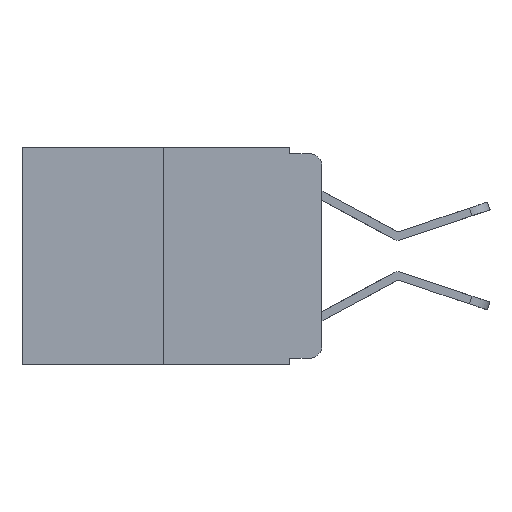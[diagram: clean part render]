
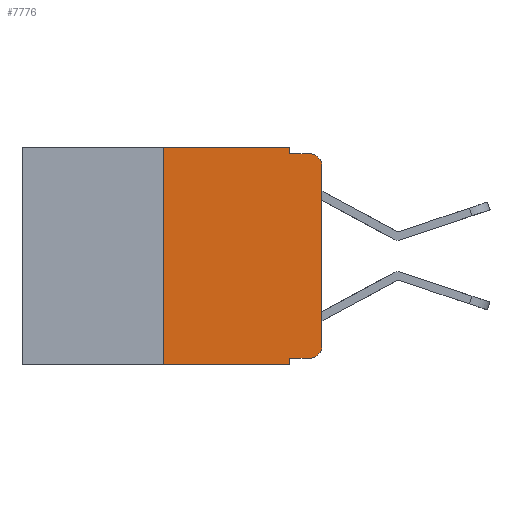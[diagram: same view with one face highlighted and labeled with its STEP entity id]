
A CAD part, left-side view. The second image highlights one B-rep face of the part: STEP entity #7776.
In plain terms, the highlighted planar face has unit normal (-1, 0, 0).
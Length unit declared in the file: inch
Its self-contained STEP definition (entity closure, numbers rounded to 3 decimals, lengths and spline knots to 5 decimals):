
#4 = DIRECTION ( 'NONE',  ( 0., 0., -1. ) ) ;
#167 = ORIENTED_EDGE ( 'NONE', *, *, #11082, .F. ) ;
#398 = CARTESIAN_POINT ( 'NONE',  ( 0., 0.051, 0. ) ) ;
#600 = VERTEX_POINT ( 'NONE', #7231 ) ;
#603 = CARTESIAN_POINT ( 'NONE',  ( 0., 0.473, 0. ) ) ;
#617 = CARTESIAN_POINT ( 'NONE',  ( 0., 0.25, -0.343 ) ) ;
#632 = VECTOR ( 'NONE', #6622, 39.37008 ) ;
#697 = ORIENTED_EDGE ( 'NONE', *, *, #9980, .F. ) ;
#709 = EDGE_CURVE ( 'NONE', #600, #5956, #1566, .T. ) ;
#1296 = CARTESIAN_POINT ( 'NONE',  ( 0., 0.051, -0.333 ) ) ;
#1396 = LINE ( 'NONE', #5989, #6309 ) ;
#1516 = VECTOR ( 'NONE', #7688, 39.37008 ) ;
#1566 = CIRCLE ( 'NONE', #11200, 0.02 ) ;
#1729 = LINE ( 'NONE', #7866, #11044 ) ;
#1887 = AXIS2_PLACEMENT_3D ( 'NONE', #603, #4783, #11041 ) ;
#2132 = AXIS2_PLACEMENT_3D ( 'NONE', #11404, #6099, #4 ) ;
#2157 = DIRECTION ( 'NONE',  ( 0., 0., -1. ) ) ;
#2173 = EDGE_CURVE ( 'NONE', #11813, #600, #6433, .T. ) ;
#2207 = LINE ( 'NONE', #9805, #11421 ) ;
#2435 = CARTESIAN_POINT ( 'NONE',  ( 0., 0.25, 0. ) ) ;
#2783 = CARTESIAN_POINT ( 'NONE',  ( 0., 0.473, 0. ) ) ;
#2790 = PLANE ( 'NONE',  #1887 ) ;
#2823 = EDGE_LOOP ( 'NONE', ( #3531, #11302, #6900, #167, #8032, #11444, #7324, #697, #4766, #12078 ) ) ;
#3334 = DIRECTION ( 'NONE',  ( 0., 0., -1. ) ) ;
#3367 = VERTEX_POINT ( 'NONE', #617 ) ;
#3529 = DIRECTION ( 'NONE',  ( 0., 0., -1. ) ) ;
#3531 = ORIENTED_EDGE ( 'NONE', *, *, #2173, .T. ) ;
#3745 = VERTEX_POINT ( 'NONE', #5617 ) ;
#3793 = LINE ( 'NONE', #2783, #632 ) ;
#4589 = VERTEX_POINT ( 'NONE', #6324 ) ;
#4712 = VERTEX_POINT ( 'NONE', #2435 ) ;
#4766 = ORIENTED_EDGE ( 'NONE', *, *, #8767, .T. ) ;
#4783 = DIRECTION ( 'NONE',  ( 1., 0., 0. ) ) ;
#5617 = CARTESIAN_POINT ( 'NONE',  ( 0., 0.051, -0.01 ) ) ;
#5956 = VERTEX_POINT ( 'NONE', #6117 ) ;
#5989 = CARTESIAN_POINT ( 'NONE',  ( 0., 0.473, -0.343 ) ) ;
#6099 = DIRECTION ( 'NONE',  ( -1., 0., 0. ) ) ;
#6117 = CARTESIAN_POINT ( 'NONE',  ( 0., 0.02, -0.01 ) ) ;
#6309 = VECTOR ( 'NONE', #12121, 39.37008 ) ;
#6317 = VECTOR ( 'NONE', #7895, 39.37008 ) ;
#6324 = CARTESIAN_POINT ( 'NONE',  ( 0., 0.02, -0.333 ) ) ;
#6433 = LINE ( 'NONE', #9968, #8572 ) ;
#6622 = DIRECTION ( 'NONE',  ( 0., -1., 0. ) ) ;
#6708 = LINE ( 'NONE', #7722, #1516 ) ;
#6770 = CARTESIAN_POINT ( 'NONE',  ( 0., 0.02, -0.03 ) ) ;
#6869 = EDGE_CURVE ( 'NONE', #3367, #8077, #1396, .T. ) ;
#6900 = ORIENTED_EDGE ( 'NONE', *, *, #12176, .F. ) ;
#7095 = CIRCLE ( 'NONE', #2132, 0.02 ) ;
#7231 = CARTESIAN_POINT ( 'NONE',  ( 0., 0., -0.03 ) ) ;
#7236 = FACE_OUTER_BOUND ( 'NONE', #2823, .T. ) ;
#7324 = ORIENTED_EDGE ( 'NONE', *, *, #6869, .T. ) ;
#7500 = VERTEX_POINT ( 'NONE', #8697 ) ;
#7547 = EDGE_CURVE ( 'NONE', #4589, #11813, #7095, .T. ) ;
#7688 = DIRECTION ( 'NONE',  ( 0., -1., 0. ) ) ;
#7722 = CARTESIAN_POINT ( 'NONE',  ( 0., 0.051, -0.01 ) ) ;
#7776 = ADVANCED_FACE ( 'NONE', ( #7236 ), #2790, .F. ) ;
#7866 = CARTESIAN_POINT ( 'NONE',  ( 0., 0.051, 0. ) ) ;
#7895 = DIRECTION ( 'NONE',  ( 0., 0., 1. ) ) ;
#7911 = VECTOR ( 'NONE', #9882, 39.37008 ) ;
#8032 = ORIENTED_EDGE ( 'NONE', *, *, #12046, .F. ) ;
#8077 = VERTEX_POINT ( 'NONE', #12187 ) ;
#8199 = LINE ( 'NONE', #1296, #7911 ) ;
#8218 = CARTESIAN_POINT ( 'NONE',  ( 0., 0., -0.313 ) ) ;
#8572 = VECTOR ( 'NONE', #9982, 39.37008 ) ;
#8697 = CARTESIAN_POINT ( 'NONE',  ( 0., 0.051, -0.333 ) ) ;
#8767 = EDGE_CURVE ( 'NONE', #7500, #4589, #8199, .T. ) ;
#9035 = LINE ( 'NONE', #12186, #6317 ) ;
#9805 = CARTESIAN_POINT ( 'NONE',  ( 0., 0.051, 0. ) ) ;
#9882 = DIRECTION ( 'NONE',  ( 0., -1., 0. ) ) ;
#9968 = CARTESIAN_POINT ( 'NONE',  ( 0., 0., 0. ) ) ;
#9980 = EDGE_CURVE ( 'NONE', #7500, #8077, #1729, .T. ) ;
#9982 = DIRECTION ( 'NONE',  ( 0., 0., 1. ) ) ;
#10557 = EDGE_CURVE ( 'NONE', #3367, #4712, #9035, .T. ) ;
#10558 = DIRECTION ( 'NONE',  ( -1., 0., 0. ) ) ;
#11041 = DIRECTION ( 'NONE',  ( 0., 0., -1. ) ) ;
#11044 = VECTOR ( 'NONE', #2157, 39.37008 ) ;
#11082 = EDGE_CURVE ( 'NONE', #11932, #3745, #2207, .T. ) ;
#11200 = AXIS2_PLACEMENT_3D ( 'NONE', #6770, #10558, #3529 ) ;
#11302 = ORIENTED_EDGE ( 'NONE', *, *, #709, .T. ) ;
#11404 = CARTESIAN_POINT ( 'NONE',  ( 0., 0.02, -0.313 ) ) ;
#11421 = VECTOR ( 'NONE', #3334, 39.37008 ) ;
#11444 = ORIENTED_EDGE ( 'NONE', *, *, #10557, .F. ) ;
#11813 = VERTEX_POINT ( 'NONE', #8218 ) ;
#11932 = VERTEX_POINT ( 'NONE', #398 ) ;
#12046 = EDGE_CURVE ( 'NONE', #4712, #11932, #3793, .T. ) ;
#12078 = ORIENTED_EDGE ( 'NONE', *, *, #7547, .T. ) ;
#12121 = DIRECTION ( 'NONE',  ( 0., -1., 0. ) ) ;
#12176 = EDGE_CURVE ( 'NONE', #3745, #5956, #6708, .T. ) ;
#12186 = CARTESIAN_POINT ( 'NONE',  ( 0., 0.25, 0. ) ) ;
#12187 = CARTESIAN_POINT ( 'NONE',  ( 0., 0.051, -0.343 ) ) ;
